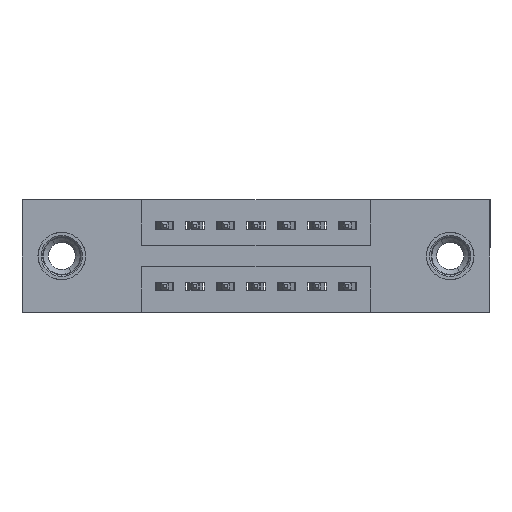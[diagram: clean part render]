
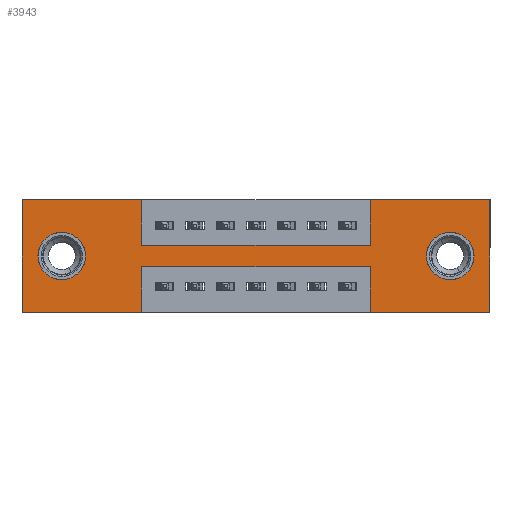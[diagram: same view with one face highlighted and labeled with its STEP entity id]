
A CAD part, front view. The second image highlights one B-rep face of the part: STEP entity #3943.
In plain terms, the highlighted planar face has unit normal (0, -1, 0).
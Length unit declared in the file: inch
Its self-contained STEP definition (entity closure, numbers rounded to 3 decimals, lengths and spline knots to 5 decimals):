
#1 = PLANE ( 'NONE',  #7085 ) ;
#74 = CARTESIAN_POINT ( 'NONE',  ( 1.405, 0., -0.185 ) ) ;
#88 = CARTESIAN_POINT ( 'NONE',  ( 0., 0., -0.37 ) ) ;
#204 = DIRECTION ( 'NONE',  ( 0., 0., 1. ) ) ;
#230 = CARTESIAN_POINT ( 'NONE',  ( 0.13, 0., -0.185 ) ) ;
#241 = CIRCLE ( 'NONE', #12201, 0.078 ) ;
#390 = CARTESIAN_POINT ( 'NONE',  ( 0., 0., -0.37 ) ) ;
#423 = LINE ( 'NONE', #5958, #8349 ) ;
#507 = CARTESIAN_POINT ( 'NONE',  ( 0.3925, 0., -0.22 ) ) ;
#540 = CARTESIAN_POINT ( 'NONE',  ( 0.3925, 0., -0.22 ) ) ;
#549 = VECTOR ( 'NONE', #4222, 39.37008 ) ;
#644 = VERTEX_POINT ( 'NONE', #11504 ) ;
#683 = AXIS2_PLACEMENT_3D ( 'NONE', #1366, #1331, #1314 ) ;
#726 = FACE_BOUND ( 'NONE', #2688, .T. ) ;
#824 = LINE ( 'NONE', #8291, #5892 ) ;
#1240 = DIRECTION ( 'NONE',  ( 0., 0., 1. ) ) ;
#1266 = EDGE_CURVE ( 'NONE', #5100, #9426, #2703, .T. ) ;
#1298 = LINE ( 'NONE', #507, #10845 ) ;
#1314 = DIRECTION ( 'NONE',  ( 0., 0., -1. ) ) ;
#1331 = DIRECTION ( 'NONE',  ( 0., 1., 0. ) ) ;
#1349 = VECTOR ( 'NONE', #5408, 39.37008 ) ;
#1366 = CARTESIAN_POINT ( 'NONE',  ( 1.405, 0., -0.185 ) ) ;
#1638 = CARTESIAN_POINT ( 'NONE',  ( 0.3925, 0., -0.15 ) ) ;
#1683 = CARTESIAN_POINT ( 'NONE',  ( 0.13, 0., -0.263 ) ) ;
#1696 = DIRECTION ( 'NONE',  ( 1., 0., 0. ) ) ;
#1713 = VERTEX_POINT ( 'NONE', #1683 ) ;
#1718 = EDGE_CURVE ( 'NONE', #9511, #11186, #5217, .T. ) ;
#1992 = CARTESIAN_POINT ( 'NONE',  ( 0.3925, 0., -0.37 ) ) ;
#2066 = EDGE_CURVE ( 'NONE', #4535, #644, #3575, .T. ) ;
#2260 = ORIENTED_EDGE ( 'NONE', *, *, #11698, .F. ) ;
#2294 = EDGE_CURVE ( 'NONE', #6398, #7939, #11014, .T. ) ;
#2396 = VECTOR ( 'NONE', #7148, 39.37008 ) ;
#2485 = ORIENTED_EDGE ( 'NONE', *, *, #2066, .T. ) ;
#2499 = CARTESIAN_POINT ( 'NONE',  ( 0.3925, 0., -0.15 ) ) ;
#2552 = DIRECTION ( 'NONE',  ( 0., 0., -1. ) ) ;
#2608 = EDGE_LOOP ( 'NONE', ( #8544, #7074 ) ) ;
#2688 = EDGE_LOOP ( 'NONE', ( #2485, #8312 ) ) ;
#2703 = LINE ( 'NONE', #9481, #2396 ) ;
#2810 = ORIENTED_EDGE ( 'NONE', *, *, #11595, .F. ) ;
#3258 = CARTESIAN_POINT ( 'NONE',  ( 0.3925, 0., 0. ) ) ;
#3495 = ORIENTED_EDGE ( 'NONE', *, *, #6403, .F. ) ;
#3527 = CARTESIAN_POINT ( 'NONE',  ( 0., 0., 0. ) ) ;
#3544 = EDGE_CURVE ( 'NONE', #9426, #6374, #6802, .T. ) ;
#3575 = CIRCLE ( 'NONE', #11309, 0.078 ) ;
#3714 = VERTEX_POINT ( 'NONE', #11276 ) ;
#3843 = ORIENTED_EDGE ( 'NONE', *, *, #1718, .F. ) ;
#3852 = EDGE_CURVE ( 'NONE', #644, #4535, #11771, .T. ) ;
#3891 = LINE ( 'NONE', #11108, #1349 ) ;
#3914 = DIRECTION ( 'NONE',  ( 0., 0., -1. ) ) ;
#3943 = ADVANCED_FACE ( 'NONE', ( #726, #8625, #10889 ), #1, .T. ) ;
#4052 = CARTESIAN_POINT ( 'NONE',  ( 0., 0., -0.37 ) ) ;
#4118 = VERTEX_POINT ( 'NONE', #9489 ) ;
#4146 = DIRECTION ( 'NONE',  ( -1., 0., 0. ) ) ;
#4174 = CARTESIAN_POINT ( 'NONE',  ( 0., 0., 0. ) ) ;
#4193 = CARTESIAN_POINT ( 'NONE',  ( 1.1425, 0., 0. ) ) ;
#4218 = DIRECTION ( 'NONE',  ( 0., 1., 0. ) ) ;
#4222 = DIRECTION ( 'NONE',  ( -1., 0., 0. ) ) ;
#4242 = EDGE_CURVE ( 'NONE', #7609, #6398, #7586, .T. ) ;
#4489 = DIRECTION ( 'NONE',  ( 0., 1., 0. ) ) ;
#4527 = DIRECTION ( 'NONE',  ( 0., 0., -1. ) ) ;
#4535 = VERTEX_POINT ( 'NONE', #7477 ) ;
#5100 = VERTEX_POINT ( 'NONE', #7298 ) ;
#5137 = ORIENTED_EDGE ( 'NONE', *, *, #2294, .F. ) ;
#5217 = LINE ( 'NONE', #1638, #12210 ) ;
#5391 = CARTESIAN_POINT ( 'NONE',  ( 1.1425, 0., -0.15 ) ) ;
#5408 = DIRECTION ( 'NONE',  ( 0., 0., 1. ) ) ;
#5442 = CARTESIAN_POINT ( 'NONE',  ( 0.3925, 0., -0.37 ) ) ;
#5630 = AXIS2_PLACEMENT_3D ( 'NONE', #9910, #4218, #10886 ) ;
#5678 = EDGE_CURVE ( 'NONE', #6742, #7609, #1298, .T. ) ;
#5884 = LINE ( 'NONE', #4174, #8406 ) ;
#5892 = VECTOR ( 'NONE', #12093, 39.37008 ) ;
#5958 = CARTESIAN_POINT ( 'NONE',  ( 1.1425, 0., -0.37 ) ) ;
#6177 = CIRCLE ( 'NONE', #5630, 0.078 ) ;
#6374 = VERTEX_POINT ( 'NONE', #12047 ) ;
#6398 = VERTEX_POINT ( 'NONE', #5442 ) ;
#6403 = EDGE_CURVE ( 'NONE', #11186, #12369, #824, .T. ) ;
#6465 = VECTOR ( 'NONE', #12095, 39.37008 ) ;
#6571 = VECTOR ( 'NONE', #10844, 39.37008 ) ;
#6742 = VERTEX_POINT ( 'NONE', #10696 ) ;
#6802 = LINE ( 'NONE', #4052, #9321 ) ;
#6841 = EDGE_CURVE ( 'NONE', #12369, #5100, #5884, .T. ) ;
#6862 = EDGE_CURVE ( 'NONE', #12228, #1713, #6177, .T. ) ;
#6941 = DIRECTION ( 'NONE',  ( 0., 1., 0. ) ) ;
#6944 = ORIENTED_EDGE ( 'NONE', *, *, #7671, .F. ) ;
#7014 = ORIENTED_EDGE ( 'NONE', *, *, #4242, .F. ) ;
#7074 = ORIENTED_EDGE ( 'NONE', *, *, #12279, .T. ) ;
#7085 = AXIS2_PLACEMENT_3D ( 'NONE', #390, #8221, #2552 ) ;
#7148 = DIRECTION ( 'NONE',  ( 0., 0., -1. ) ) ;
#7201 = DIRECTION ( 'NONE',  ( -1., 0., 0. ) ) ;
#7288 = VECTOR ( 'NONE', #3914, 39.37008 ) ;
#7298 = CARTESIAN_POINT ( 'NONE',  ( 1.535, 0., 0. ) ) ;
#7422 = ORIENTED_EDGE ( 'NONE', *, *, #9546, .F. ) ;
#7477 = CARTESIAN_POINT ( 'NONE',  ( 1.405, 0., -0.107 ) ) ;
#7586 = LINE ( 'NONE', #1992, #7288 ) ;
#7609 = VERTEX_POINT ( 'NONE', #540 ) ;
#7671 = EDGE_CURVE ( 'NONE', #4118, #3714, #11820, .T. ) ;
#7868 = ORIENTED_EDGE ( 'NONE', *, *, #6841, .F. ) ;
#7939 = VERTEX_POINT ( 'NONE', #88 ) ;
#8221 = DIRECTION ( 'NONE',  ( 0., -1., 0. ) ) ;
#8291 = CARTESIAN_POINT ( 'NONE',  ( 1.1425, 0., 0. ) ) ;
#8312 = ORIENTED_EDGE ( 'NONE', *, *, #3852, .T. ) ;
#8349 = VECTOR ( 'NONE', #204, 39.37008 ) ;
#8406 = VECTOR ( 'NONE', #8902, 39.37008 ) ;
#8544 = ORIENTED_EDGE ( 'NONE', *, *, #6862, .T. ) ;
#8545 = ORIENTED_EDGE ( 'NONE', *, *, #1266, .F. ) ;
#8556 = CARTESIAN_POINT ( 'NONE',  ( 0., 0., -0.37 ) ) ;
#8625 = FACE_BOUND ( 'NONE', #2608, .T. ) ;
#8902 = DIRECTION ( 'NONE',  ( 1., 0., 0. ) ) ;
#9081 = LINE ( 'NONE', #3258, #6571 ) ;
#9257 = ORIENTED_EDGE ( 'NONE', *, *, #3544, .F. ) ;
#9321 = VECTOR ( 'NONE', #4146, 39.37008 ) ;
#9426 = VERTEX_POINT ( 'NONE', #10949 ) ;
#9481 = CARTESIAN_POINT ( 'NONE',  ( 1.535, 0., 0. ) ) ;
#9489 = CARTESIAN_POINT ( 'NONE',  ( 0., 0., 0. ) ) ;
#9511 = VERTEX_POINT ( 'NONE', #2499 ) ;
#9546 = EDGE_CURVE ( 'NONE', #7939, #4118, #3891, .T. ) ;
#9910 = CARTESIAN_POINT ( 'NONE',  ( 0.13, 0., -0.185 ) ) ;
#10436 = EDGE_LOOP ( 'NONE', ( #7014, #10642, #2810, #9257, #8545, #7868, #3495, #3843, #2260, #6944, #7422, #5137 ) ) ;
#10642 = ORIENTED_EDGE ( 'NONE', *, *, #5678, .F. ) ;
#10668 = CARTESIAN_POINT ( 'NONE',  ( 0.13, 0., -0.107 ) ) ;
#10696 = CARTESIAN_POINT ( 'NONE',  ( 1.1425, 0., -0.22 ) ) ;
#10844 = DIRECTION ( 'NONE',  ( 0., 0., -1. ) ) ;
#10845 = VECTOR ( 'NONE', #7201, 39.37008 ) ;
#10886 = DIRECTION ( 'NONE',  ( 0., 0., 1. ) ) ;
#10889 = FACE_OUTER_BOUND ( 'NONE', #10436, .T. ) ;
#10949 = CARTESIAN_POINT ( 'NONE',  ( 1.535, 0., -0.37 ) ) ;
#11014 = LINE ( 'NONE', #8556, #549 ) ;
#11108 = CARTESIAN_POINT ( 'NONE',  ( 0., 0., 0. ) ) ;
#11186 = VERTEX_POINT ( 'NONE', #5391 ) ;
#11276 = CARTESIAN_POINT ( 'NONE',  ( 0.3925, 0., 0. ) ) ;
#11309 = AXIS2_PLACEMENT_3D ( 'NONE', #74, #4489, #4527 ) ;
#11504 = CARTESIAN_POINT ( 'NONE',  ( 1.405, 0., -0.263 ) ) ;
#11595 = EDGE_CURVE ( 'NONE', #6374, #6742, #423, .T. ) ;
#11698 = EDGE_CURVE ( 'NONE', #3714, #9511, #9081, .T. ) ;
#11771 = CIRCLE ( 'NONE', #683, 0.078 ) ;
#11820 = LINE ( 'NONE', #3527, #6465 ) ;
#12047 = CARTESIAN_POINT ( 'NONE',  ( 1.1425, 0., -0.37 ) ) ;
#12093 = DIRECTION ( 'NONE',  ( 0., 0., 1. ) ) ;
#12095 = DIRECTION ( 'NONE',  ( 1., 0., 0. ) ) ;
#12201 = AXIS2_PLACEMENT_3D ( 'NONE', #230, #6941, #1240 ) ;
#12210 = VECTOR ( 'NONE', #1696, 39.37008 ) ;
#12228 = VERTEX_POINT ( 'NONE', #10668 ) ;
#12279 = EDGE_CURVE ( 'NONE', #1713, #12228, #241, .T. ) ;
#12369 = VERTEX_POINT ( 'NONE', #4193 ) ;
